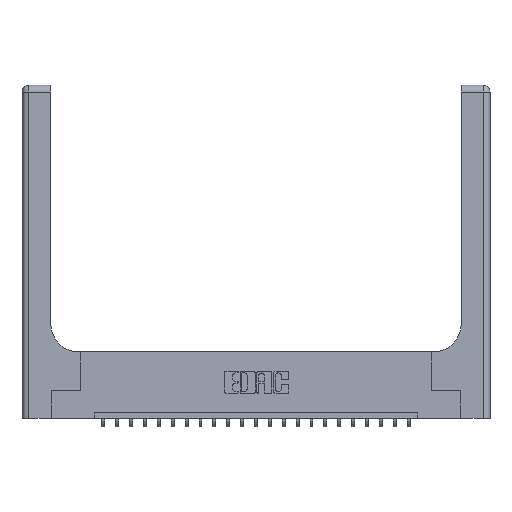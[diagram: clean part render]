
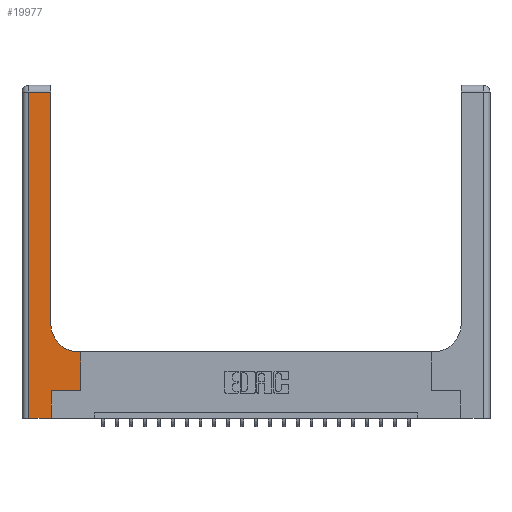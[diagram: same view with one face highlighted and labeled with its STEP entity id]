
A CAD part, top view. The second image highlights one B-rep face of the part: STEP entity #19977.
In plain terms, the highlighted planar face has unit normal (0, 0, 1).
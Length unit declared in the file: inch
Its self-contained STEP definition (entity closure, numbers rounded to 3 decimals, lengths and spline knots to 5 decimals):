
#88 = DIRECTION ( 'NONE',  ( 1., 0., 0. ) ) ;
#638 = CARTESIAN_POINT ( 'NONE',  ( 0.26, 0.85, 0.37 ) ) ;
#736 = VECTOR ( 'NONE', #16974, 39.37008 ) ;
#836 = VECTOR ( 'NONE', #8550, 39.37008 ) ;
#1029 = VERTEX_POINT ( 'NONE', #638 ) ;
#1238 = VERTEX_POINT ( 'NONE', #8819 ) ;
#1269 = CARTESIAN_POINT ( 'NONE',  ( 0., 3., 0.37 ) ) ;
#1948 = EDGE_CURVE ( 'NONE', #1238, #1029, #4598, .T. ) ;
#2432 = VERTEX_POINT ( 'NONE', #6782 ) ;
#2562 = VECTOR ( 'NONE', #16713, 39.37008 ) ;
#2726 = VERTEX_POINT ( 'NONE', #11546 ) ;
#3059 = EDGE_CURVE ( 'NONE', #2432, #16704, #20070, .T. ) ;
#3325 = DIRECTION ( 'NONE',  ( 0., 0., -1. ) ) ;
#4070 = EDGE_LOOP ( 'NONE', ( #9487, #10477, #17933, #16141, #10812, #4265, #21727, #7430, #10158 ) ) ;
#4265 = ORIENTED_EDGE ( 'NONE', *, *, #17080, .T. ) ;
#4459 = CARTESIAN_POINT ( 'NONE',  ( 0.26, 3., 0.37 ) ) ;
#4598 = CIRCLE ( 'NONE', #19545, 0.25 ) ;
#4688 = LINE ( 'NONE', #22243, #16007 ) ;
#4973 = CARTESIAN_POINT ( 'NONE',  ( 0.528, 0.6, 0.37 ) ) ;
#6166 = DIRECTION ( 'NONE',  ( 1., 0., 0. ) ) ;
#6277 = LINE ( 'NONE', #4459, #6950 ) ;
#6629 = EDGE_CURVE ( 'NONE', #17059, #1238, #20503, .T. ) ;
#6782 = CARTESIAN_POINT ( 'NONE',  ( 0.06, 0., 0.37 ) ) ;
#6950 = VECTOR ( 'NONE', #20308, 39.37008 ) ;
#7430 = ORIENTED_EDGE ( 'NONE', *, *, #6629, .T. ) ;
#8040 = LINE ( 'NONE', #16599, #2562 ) ;
#8212 = DIRECTION ( 'NONE',  ( -1., 0., 0. ) ) ;
#8550 = DIRECTION ( 'NONE',  ( 0., -1., 0. ) ) ;
#8819 = CARTESIAN_POINT ( 'NONE',  ( 0.51, 0.6, 0.37 ) ) ;
#9166 = CARTESIAN_POINT ( 'NONE',  ( 0.528, 0.25, 0.37 ) ) ;
#9487 = ORIENTED_EDGE ( 'NONE', *, *, #17976, .T. ) ;
#10158 = ORIENTED_EDGE ( 'NONE', *, *, #1948, .T. ) ;
#10477 = ORIENTED_EDGE ( 'NONE', *, *, #16386, .T. ) ;
#10812 = ORIENTED_EDGE ( 'NONE', *, *, #18848, .T. ) ;
#10891 = CARTESIAN_POINT ( 'NONE',  ( 0.06, 2.94, 0.37 ) ) ;
#11289 = CARTESIAN_POINT ( 'NONE',  ( 0., 0., 0.37 ) ) ;
#11546 = CARTESIAN_POINT ( 'NONE',  ( 0.265, 0.25, 0.37 ) ) ;
#11644 = PLANE ( 'NONE',  #21227 ) ;
#13686 = LINE ( 'NONE', #15295, #836 ) ;
#14145 = VERTEX_POINT ( 'NONE', #21230 ) ;
#15295 = CARTESIAN_POINT ( 'NONE',  ( 0.06, 3., 0.37 ) ) ;
#15321 = LINE ( 'NONE', #22277, #19722 ) ;
#15364 = CARTESIAN_POINT ( 'NONE',  ( 0.51, 0.85, 0.37 ) ) ;
#15481 = CARTESIAN_POINT ( 'NONE',  ( 0.265, 0., 0.37 ) ) ;
#16007 = VECTOR ( 'NONE', #18933, 39.37008 ) ;
#16141 = ORIENTED_EDGE ( 'NONE', *, *, #3059, .T. ) ;
#16386 = EDGE_CURVE ( 'NONE', #14145, #21869, #4688, .T. ) ;
#16599 = CARTESIAN_POINT ( 'NONE',  ( 0.265, 0.25, 0.37 ) ) ;
#16704 = VERTEX_POINT ( 'NONE', #15481 ) ;
#16713 = DIRECTION ( 'NONE',  ( 1., 0., 0. ) ) ;
#16974 = DIRECTION ( 'NONE',  ( -1., 0., 0. ) ) ;
#17059 = VERTEX_POINT ( 'NONE', #4973 ) ;
#17071 = DIRECTION ( 'NONE',  ( 0., 0., -1. ) ) ;
#17080 = EDGE_CURVE ( 'NONE', #2726, #22195, #8040, .T. ) ;
#17933 = ORIENTED_EDGE ( 'NONE', *, *, #19987, .T. ) ;
#17976 = EDGE_CURVE ( 'NONE', #1029, #14145, #6277, .T. ) ;
#18459 = CARTESIAN_POINT ( 'NONE',  ( 0.26, 0.6, 0.37 ) ) ;
#18598 = EDGE_CURVE ( 'NONE', #22195, #17059, #21711, .T. ) ;
#18848 = EDGE_CURVE ( 'NONE', #16704, #2726, #15321, .T. ) ;
#18933 = DIRECTION ( 'NONE',  ( -1., 0., 0. ) ) ;
#19545 = AXIS2_PLACEMENT_3D ( 'NONE', #15364, #17071, #88 ) ;
#19655 = DIRECTION ( 'NONE',  ( 0., 1., 0. ) ) ;
#19722 = VECTOR ( 'NONE', #20109, 39.37008 ) ;
#19977 = ADVANCED_FACE ( 'NONE', ( #22253 ), #11644, .F. ) ;
#19987 = EDGE_CURVE ( 'NONE', #21869, #2432, #13686, .T. ) ;
#20070 = LINE ( 'NONE', #11289, #20079 ) ;
#20079 = VECTOR ( 'NONE', #6166, 39.37008 ) ;
#20109 = DIRECTION ( 'NONE',  ( 0., 1., 0. ) ) ;
#20233 = CARTESIAN_POINT ( 'NONE',  ( 0.528, 0.25, 0.37 ) ) ;
#20308 = DIRECTION ( 'NONE',  ( 0., 1., 0. ) ) ;
#20503 = LINE ( 'NONE', #18459, #736 ) ;
#21227 = AXIS2_PLACEMENT_3D ( 'NONE', #1269, #3325, #8212 ) ;
#21230 = CARTESIAN_POINT ( 'NONE',  ( 0.26, 2.94, 0.37 ) ) ;
#21711 = LINE ( 'NONE', #9166, #21909 ) ;
#21727 = ORIENTED_EDGE ( 'NONE', *, *, #18598, .T. ) ;
#21869 = VERTEX_POINT ( 'NONE', #10891 ) ;
#21909 = VECTOR ( 'NONE', #19655, 39.37008 ) ;
#22195 = VERTEX_POINT ( 'NONE', #20233 ) ;
#22243 = CARTESIAN_POINT ( 'NONE',  ( 0., 2.94, 0.37 ) ) ;
#22253 = FACE_OUTER_BOUND ( 'NONE', #4070, .T. ) ;
#22277 = CARTESIAN_POINT ( 'NONE',  ( 0.265, 0., 0.37 ) ) ;
